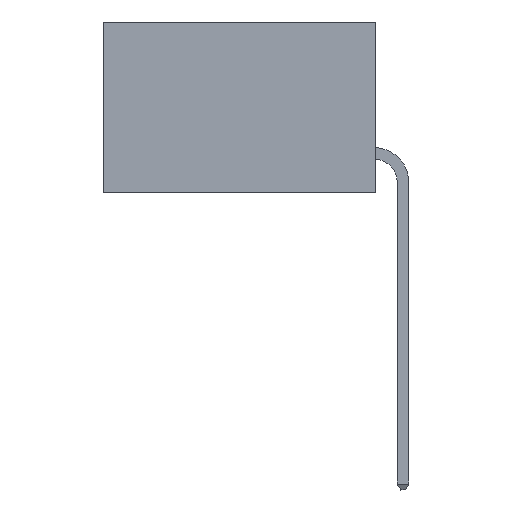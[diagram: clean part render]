
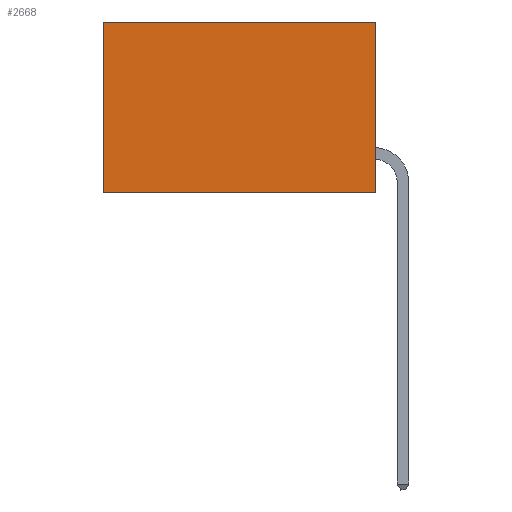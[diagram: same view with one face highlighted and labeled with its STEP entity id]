
A CAD part, left-side view. The second image highlights one B-rep face of the part: STEP entity #2668.
In plain terms, the highlighted planar face has unit normal (-1, 0, 0).
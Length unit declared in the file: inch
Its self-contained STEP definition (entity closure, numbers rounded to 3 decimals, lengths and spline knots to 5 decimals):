
#772 = CARTESIAN_POINT ( 'NONE',  ( 0.277, 0., -0.37 ) ) ;
#839 = LINE ( 'NONE', #1162, #5333 ) ;
#883 = DIRECTION ( 'NONE',  ( 0., 0., -1. ) ) ;
#1162 = CARTESIAN_POINT ( 'NONE',  ( 0.277, 0., -0.37 ) ) ;
#1400 = CARTESIAN_POINT ( 'NONE',  ( 0.277, 0.59, 0. ) ) ;
#2191 = CARTESIAN_POINT ( 'NONE',  ( 0.277, 0.59, -0.37 ) ) ;
#2668 = ADVANCED_FACE ( 'NONE', ( #13943 ), #9328, .F. ) ;
#2745 = CARTESIAN_POINT ( 'NONE',  ( 0.277, 0., 0. ) ) ;
#5036 = CARTESIAN_POINT ( 'NONE',  ( 0.277, 0., -0.37 ) ) ;
#5333 = VECTOR ( 'NONE', #16663, 39.37008 ) ;
#6331 = EDGE_LOOP ( 'NONE', ( #8768, #24811, #7063, #10296 ) ) ;
#6548 = VERTEX_POINT ( 'NONE', #1400 ) ;
#7063 = ORIENTED_EDGE ( 'NONE', *, *, #27225, .F. ) ;
#8768 = ORIENTED_EDGE ( 'NONE', *, *, #16070, .T. ) ;
#9328 = PLANE ( 'NONE',  #26811 ) ;
#9833 = EDGE_CURVE ( 'NONE', #20894, #16742, #24249, .T. ) ;
#10296 = ORIENTED_EDGE ( 'NONE', *, *, #15300, .T. ) ;
#12117 = LINE ( 'NONE', #29652, #24815 ) ;
#13943 = FACE_OUTER_BOUND ( 'NONE', #6331, .T. ) ;
#14873 = VERTEX_POINT ( 'NONE', #2745 ) ;
#15300 = EDGE_CURVE ( 'NONE', #14873, #6548, #12117, .T. ) ;
#16070 = EDGE_CURVE ( 'NONE', #6548, #16742, #21267, .T. ) ;
#16663 = DIRECTION ( 'NONE',  ( 0., 0., -1. ) ) ;
#16742 = VERTEX_POINT ( 'NONE', #2191 ) ;
#16943 = DIRECTION ( 'NONE',  ( 0., 1., 0. ) ) ;
#20892 = CARTESIAN_POINT ( 'NONE',  ( 0.277, 0., -0.37 ) ) ;
#20894 = VERTEX_POINT ( 'NONE', #5036 ) ;
#21267 = LINE ( 'NONE', #28016, #27046 ) ;
#24155 = DIRECTION ( 'NONE',  ( 1., 0., 0. ) ) ;
#24249 = LINE ( 'NONE', #20892, #29267 ) ;
#24416 = DIRECTION ( 'NONE',  ( 0., 1., 0. ) ) ;
#24811 = ORIENTED_EDGE ( 'NONE', *, *, #9833, .F. ) ;
#24815 = VECTOR ( 'NONE', #16943, 39.37008 ) ;
#26811 = AXIS2_PLACEMENT_3D ( 'NONE', #772, #24155, #883 ) ;
#27046 = VECTOR ( 'NONE', #27840, 39.37008 ) ;
#27225 = EDGE_CURVE ( 'NONE', #14873, #20894, #839, .T. ) ;
#27840 = DIRECTION ( 'NONE',  ( 0., 0., -1. ) ) ;
#28016 = CARTESIAN_POINT ( 'NONE',  ( 0.277, 0.59, -0.37 ) ) ;
#29267 = VECTOR ( 'NONE', #24416, 39.37008 ) ;
#29652 = CARTESIAN_POINT ( 'NONE',  ( 0.277, 0., 0. ) ) ;
